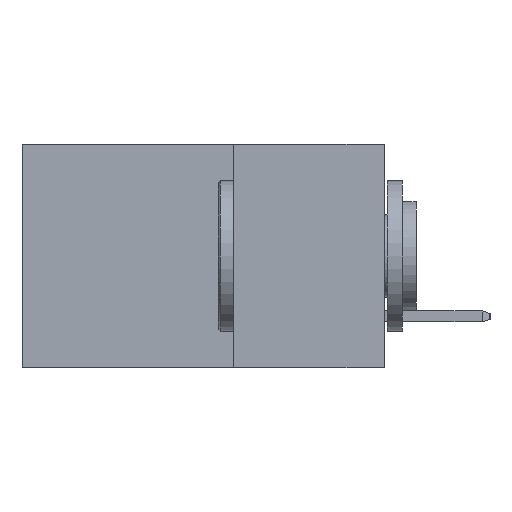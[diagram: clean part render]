
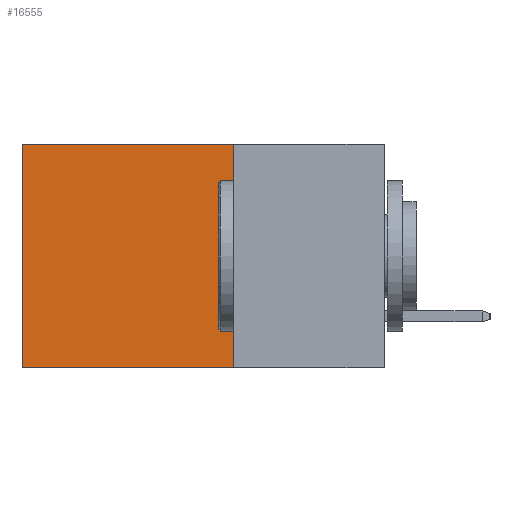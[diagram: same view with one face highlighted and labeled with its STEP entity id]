
A CAD part, left-side view. The second image highlights one B-rep face of the part: STEP entity #16555.
In plain terms, the highlighted planar face has unit normal (-1, 0, 0).
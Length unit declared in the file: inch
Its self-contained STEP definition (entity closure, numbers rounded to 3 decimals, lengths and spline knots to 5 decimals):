
#1354 = PLANE ( 'NONE',  #15614 ) ;
#1604 = EDGE_CURVE ( 'NONE', #22606, #25362, #10279, .T. ) ;
#2912 = VECTOR ( 'NONE', #18871, 39.37008 ) ;
#3041 = VERTEX_POINT ( 'NONE', #24514 ) ;
#3374 = DIRECTION ( 'NONE',  ( 0., 0., -1. ) ) ;
#3620 = CARTESIAN_POINT ( 'NONE',  ( 0.2615, 0.25, -0.37 ) ) ;
#3655 = LINE ( 'NONE', #4836, #19251 ) ;
#4836 = CARTESIAN_POINT ( 'NONE',  ( 0.2615, 0.6, -0.37 ) ) ;
#4855 = VECTOR ( 'NONE', #6818, 39.37008 ) ;
#5108 = ORIENTED_EDGE ( 'NONE', *, *, #19957, .T. ) ;
#5629 = DIRECTION ( 'NONE',  ( 0., 1., 0. ) ) ;
#6818 = DIRECTION ( 'NONE',  ( 0., 0., -1. ) ) ;
#6873 = DIRECTION ( 'NONE',  ( 0., 0., -1. ) ) ;
#7653 = VERTEX_POINT ( 'NONE', #20738 ) ;
#8043 = VECTOR ( 'NONE', #5629, 39.37008 ) ;
#8220 = EDGE_LOOP ( 'NONE', ( #5108, #8462, #26316, #25556 ) ) ;
#8249 = LINE ( 'NONE', #10656, #2912 ) ;
#8462 = ORIENTED_EDGE ( 'NONE', *, *, #20223, .F. ) ;
#8682 = LINE ( 'NONE', #3620, #8043 ) ;
#10279 = LINE ( 'NONE', #20321, #4855 ) ;
#10656 = CARTESIAN_POINT ( 'NONE',  ( 0.2615, 0.25, 0. ) ) ;
#11320 = CARTESIAN_POINT ( 'NONE',  ( 0.2615, 0.25, -0.37 ) ) ;
#14360 = CARTESIAN_POINT ( 'NONE',  ( 0.2615, 0.25, 0. ) ) ;
#15459 = CARTESIAN_POINT ( 'NONE',  ( 0.2615, 0.25, -0.37 ) ) ;
#15544 = DIRECTION ( 'NONE',  ( 1., 0., 0. ) ) ;
#15614 = AXIS2_PLACEMENT_3D ( 'NONE', #15459, #15544, #3374 ) ;
#16307 = EDGE_CURVE ( 'NONE', #22606, #7653, #8249, .T. ) ;
#16555 = ADVANCED_FACE ( 'NONE', ( #17520 ), #1354, .F. ) ;
#17520 = FACE_OUTER_BOUND ( 'NONE', #8220, .T. ) ;
#18871 = DIRECTION ( 'NONE',  ( 0., 1., 0. ) ) ;
#19251 = VECTOR ( 'NONE', #6873, 39.37008 ) ;
#19957 = EDGE_CURVE ( 'NONE', #7653, #3041, #3655, .T. ) ;
#20223 = EDGE_CURVE ( 'NONE', #25362, #3041, #8682, .T. ) ;
#20321 = CARTESIAN_POINT ( 'NONE',  ( 0.2615, 0.25, -0.37 ) ) ;
#20738 = CARTESIAN_POINT ( 'NONE',  ( 0.2615, 0.6, 0. ) ) ;
#22606 = VERTEX_POINT ( 'NONE', #14360 ) ;
#24514 = CARTESIAN_POINT ( 'NONE',  ( 0.2615, 0.6, -0.37 ) ) ;
#25362 = VERTEX_POINT ( 'NONE', #11320 ) ;
#25556 = ORIENTED_EDGE ( 'NONE', *, *, #16307, .T. ) ;
#26316 = ORIENTED_EDGE ( 'NONE', *, *, #1604, .F. ) ;
